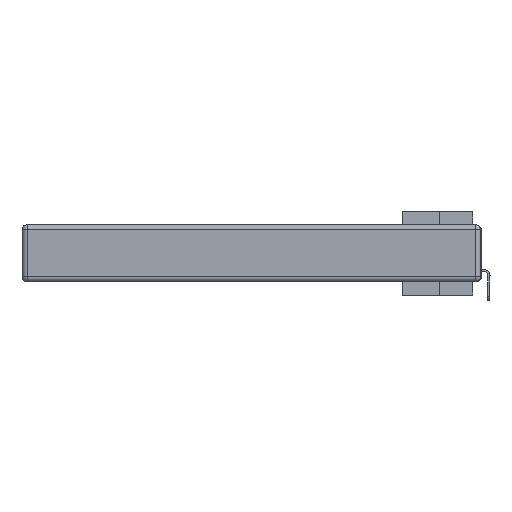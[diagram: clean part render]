
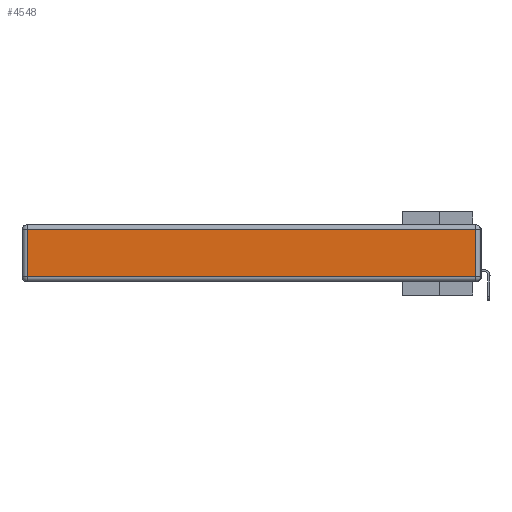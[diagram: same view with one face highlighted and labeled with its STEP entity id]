
A CAD part, left-side view. The second image highlights one B-rep face of the part: STEP entity #4548.
In plain terms, the highlighted planar face has unit normal (-1, 0, 0).
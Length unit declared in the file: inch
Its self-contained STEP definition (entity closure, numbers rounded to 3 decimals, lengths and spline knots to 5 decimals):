
#348 = CARTESIAN_POINT ( 'NONE',  ( 0., 0.03, -0.313 ) ) ;
#590 = VERTEX_POINT ( 'NONE', #348 ) ;
#1088 = FACE_OUTER_BOUND ( 'NONE', #21402, .T. ) ;
#1312 = EDGE_CURVE ( 'NONE', #19539, #590, #37177, .T. ) ;
#3347 = EDGE_CURVE ( 'NONE', #12885, #4920, #15914, .T. ) ;
#3946 = CARTESIAN_POINT ( 'NONE',  ( 0., 0.03, -0.03 ) ) ;
#4548 = ADVANCED_FACE ( 'NONE', ( #1088 ), #23240, .T. ) ;
#4568 = LINE ( 'NONE', #6861, #23974 ) ;
#4920 = VERTEX_POINT ( 'NONE', #9009 ) ;
#6656 = DIRECTION ( 'NONE',  ( 0., 1., 0. ) ) ;
#6861 = CARTESIAN_POINT ( 'NONE',  ( 0., 0.03, -0.343 ) ) ;
#7241 = ORIENTED_EDGE ( 'NONE', *, *, #24590, .T. ) ;
#7529 = LINE ( 'NONE', #19079, #8410 ) ;
#7656 = DIRECTION ( 'NONE',  ( 0., -1., 0. ) ) ;
#8410 = VECTOR ( 'NONE', #15875, 39.37008 ) ;
#8860 = DIRECTION ( 'NONE',  ( 0., 0., 1. ) ) ;
#9009 = CARTESIAN_POINT ( 'NONE',  ( 0., 2.72, -0.03 ) ) ;
#12284 = DIRECTION ( 'NONE',  ( -1., 0., 0. ) ) ;
#12885 = VERTEX_POINT ( 'NONE', #3946 ) ;
#15133 = VECTOR ( 'NONE', #6656, 39.37008 ) ;
#15140 = CARTESIAN_POINT ( 'NONE',  ( 0., 2.72, -0.313 ) ) ;
#15875 = DIRECTION ( 'NONE',  ( 0., 0., -1. ) ) ;
#15914 = LINE ( 'NONE', #18390, #15133 ) ;
#18390 = CARTESIAN_POINT ( 'NONE',  ( 0., 2.75, -0.03 ) ) ;
#19079 = CARTESIAN_POINT ( 'NONE',  ( 0., 2.72, -0.343 ) ) ;
#19539 = VERTEX_POINT ( 'NONE', #15140 ) ;
#21402 = EDGE_LOOP ( 'NONE', ( #34385, #35610, #29606, #7241 ) ) ;
#22133 = EDGE_CURVE ( 'NONE', #590, #12885, #4568, .T. ) ;
#23240 = PLANE ( 'NONE',  #35205 ) ;
#23974 = VECTOR ( 'NONE', #32975, 39.37008 ) ;
#24590 = EDGE_CURVE ( 'NONE', #4920, #19539, #7529, .T. ) ;
#25438 = CARTESIAN_POINT ( 'NONE',  ( 0., 0., -0.313 ) ) ;
#29606 = ORIENTED_EDGE ( 'NONE', *, *, #3347, .T. ) ;
#32975 = DIRECTION ( 'NONE',  ( 0., 0., 1. ) ) ;
#34385 = ORIENTED_EDGE ( 'NONE', *, *, #1312, .T. ) ;
#34805 = CARTESIAN_POINT ( 'NONE',  ( 0., 0., -0.343 ) ) ;
#35205 = AXIS2_PLACEMENT_3D ( 'NONE', #34805, #12284, #8860 ) ;
#35495 = VECTOR ( 'NONE', #7656, 39.37008 ) ;
#35610 = ORIENTED_EDGE ( 'NONE', *, *, #22133, .T. ) ;
#37177 = LINE ( 'NONE', #25438, #35495 ) ;
